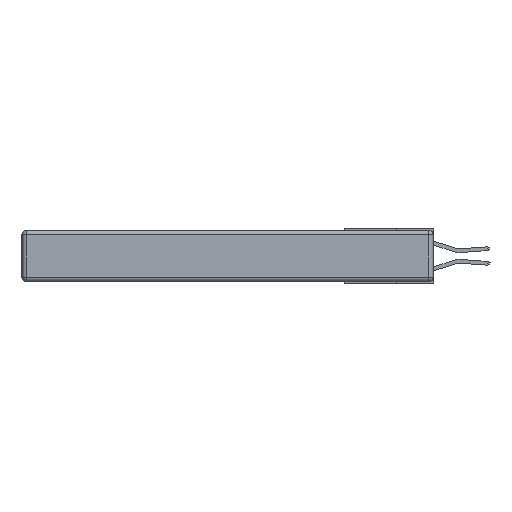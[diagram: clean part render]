
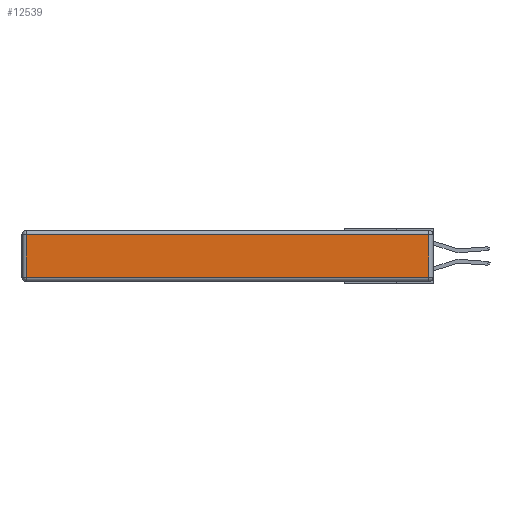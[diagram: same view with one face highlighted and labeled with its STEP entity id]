
A CAD part, left-side view. The second image highlights one B-rep face of the part: STEP entity #12539.
In plain terms, the highlighted planar face has unit normal (-1, 0, 0).
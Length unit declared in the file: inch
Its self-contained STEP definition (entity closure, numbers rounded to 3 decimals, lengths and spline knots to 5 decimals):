
#1421 = VECTOR ( 'NONE', #9475, 39.37008 ) ;
#2045 = CARTESIAN_POINT ( 'NONE',  ( 0., 2.72, -0.313 ) ) ;
#2350 = EDGE_CURVE ( 'NONE', #12595, #5733, #7783, .T. ) ;
#2415 = CARTESIAN_POINT ( 'NONE',  ( 0., 2.75, -0.03 ) ) ;
#2554 = ORIENTED_EDGE ( 'NONE', *, *, #2350, .T. ) ;
#2879 = CARTESIAN_POINT ( 'NONE',  ( 0., 0., -0.343 ) ) ;
#2938 = PLANE ( 'NONE',  #4003 ) ;
#3841 = EDGE_LOOP ( 'NONE', ( #18248, #9261, #2554, #10146 ) ) ;
#3976 = CARTESIAN_POINT ( 'NONE',  ( 0., 2.72, -0.03 ) ) ;
#4003 = AXIS2_PLACEMENT_3D ( 'NONE', #2879, #10145, #10081 ) ;
#4935 = CARTESIAN_POINT ( 'NONE',  ( 0., 0., -0.313 ) ) ;
#5576 = VECTOR ( 'NONE', #16101, 39.37008 ) ;
#5733 = VERTEX_POINT ( 'NONE', #3976 ) ;
#5745 = VECTOR ( 'NONE', #17056, 39.37008 ) ;
#6025 = CARTESIAN_POINT ( 'NONE',  ( 0., 0.03, -0.343 ) ) ;
#6419 = VECTOR ( 'NONE', #16096, 39.37008 ) ;
#7592 = EDGE_CURVE ( 'NONE', #11575, #17810, #18065, .T. ) ;
#7783 = LINE ( 'NONE', #2415, #5745 ) ;
#8530 = LINE ( 'NONE', #16226, #5576 ) ;
#9261 = ORIENTED_EDGE ( 'NONE', *, *, #17738, .T. ) ;
#9475 = DIRECTION ( 'NONE',  ( 0., -1., 0. ) ) ;
#10081 = DIRECTION ( 'NONE',  ( 0., 0., 1. ) ) ;
#10145 = DIRECTION ( 'NONE',  ( -1., 0., 0. ) ) ;
#10146 = ORIENTED_EDGE ( 'NONE', *, *, #15552, .T. ) ;
#10251 = LINE ( 'NONE', #6025, #6419 ) ;
#10834 = CARTESIAN_POINT ( 'NONE',  ( 0., 0.03, -0.313 ) ) ;
#11575 = VERTEX_POINT ( 'NONE', #2045 ) ;
#12539 = ADVANCED_FACE ( 'NONE', ( #16962 ), #2938, .T. ) ;
#12595 = VERTEX_POINT ( 'NONE', #13009 ) ;
#13009 = CARTESIAN_POINT ( 'NONE',  ( 0., 0.03, -0.03 ) ) ;
#15552 = EDGE_CURVE ( 'NONE', #5733, #11575, #8530, .T. ) ;
#16096 = DIRECTION ( 'NONE',  ( 0., 0., 1. ) ) ;
#16101 = DIRECTION ( 'NONE',  ( 0., 0., -1. ) ) ;
#16226 = CARTESIAN_POINT ( 'NONE',  ( 0., 2.72, -0.343 ) ) ;
#16962 = FACE_OUTER_BOUND ( 'NONE', #3841, .T. ) ;
#17056 = DIRECTION ( 'NONE',  ( 0., 1., 0. ) ) ;
#17738 = EDGE_CURVE ( 'NONE', #17810, #12595, #10251, .T. ) ;
#17810 = VERTEX_POINT ( 'NONE', #10834 ) ;
#18065 = LINE ( 'NONE', #4935, #1421 ) ;
#18248 = ORIENTED_EDGE ( 'NONE', *, *, #7592, .T. ) ;
